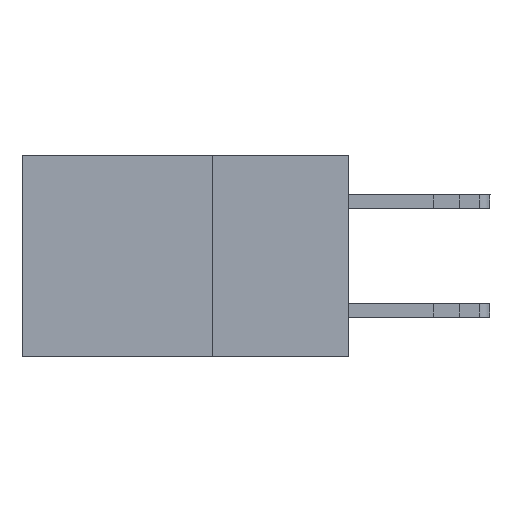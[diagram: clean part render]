
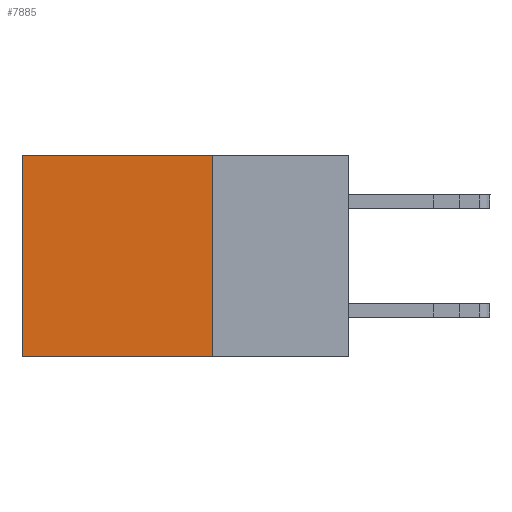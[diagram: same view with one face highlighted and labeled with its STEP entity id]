
A CAD part, left-side view. The second image highlights one B-rep face of the part: STEP entity #7885.
In plain terms, the highlighted planar face has unit normal (-1, 0, 0).
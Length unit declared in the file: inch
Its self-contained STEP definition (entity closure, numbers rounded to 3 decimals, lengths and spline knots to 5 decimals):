
#1 = CARTESIAN_POINT ( 'NONE',  ( 0.298, 0.6, 0. ) ) ;
#1360 = DIRECTION ( 'NONE',  ( 0., 0., -1. ) ) ;
#1648 = DIRECTION ( 'NONE',  ( 0., 0., -1. ) ) ;
#1945 = DIRECTION ( 'NONE',  ( 0., 0., -1. ) ) ;
#3186 = ORIENTED_EDGE ( 'NONE', *, *, #13528, .T. ) ;
#3212 = EDGE_CURVE ( 'NONE', #13332, #5409, #4690, .T. ) ;
#3219 = ORIENTED_EDGE ( 'NONE', *, *, #3212, .F. ) ;
#3785 = DIRECTION ( 'NONE',  ( 0., 1., 0. ) ) ;
#4531 = CARTESIAN_POINT ( 'NONE',  ( 0.298, 0.25, -0.37 ) ) ;
#4690 = LINE ( 'NONE', #11359, #9001 ) ;
#5409 = VERTEX_POINT ( 'NONE', #10916 ) ;
#6445 = CARTESIAN_POINT ( 'NONE',  ( 0.298, 0.6, 0. ) ) ;
#7378 = CARTESIAN_POINT ( 'NONE',  ( 0.298, 0.25, 0. ) ) ;
#7885 = ADVANCED_FACE ( 'NONE', ( #17855 ), #12615, .F. ) ;
#8250 = EDGE_LOOP ( 'NONE', ( #17135, #3219, #12923, #3186 ) ) ;
#8808 = VECTOR ( 'NONE', #1945, 39.37008 ) ;
#9001 = VECTOR ( 'NONE', #18022, 39.37008 ) ;
#9325 = EDGE_CURVE ( 'NONE', #12224, #13332, #16624, .T. ) ;
#10916 = CARTESIAN_POINT ( 'NONE',  ( 0.298, 0.6, -0.37 ) ) ;
#11359 = CARTESIAN_POINT ( 'NONE',  ( 0.298, 0.25, -0.37 ) ) ;
#11376 = CARTESIAN_POINT ( 'NONE',  ( 0.298, 0.25, 0. ) ) ;
#12224 = VERTEX_POINT ( 'NONE', #15563 ) ;
#12615 = PLANE ( 'NONE',  #15096 ) ;
#12923 = ORIENTED_EDGE ( 'NONE', *, *, #9325, .F. ) ;
#13332 = VERTEX_POINT ( 'NONE', #4531 ) ;
#13528 = EDGE_CURVE ( 'NONE', #12224, #17185, #19178, .T. ) ;
#13882 = VECTOR ( 'NONE', #3785, 39.37008 ) ;
#15096 = AXIS2_PLACEMENT_3D ( 'NONE', #19276, #17635, #1360 ) ;
#15563 = CARTESIAN_POINT ( 'NONE',  ( 0.298, 0.25, 0. ) ) ;
#16624 = LINE ( 'NONE', #11376, #19000 ) ;
#17135 = ORIENTED_EDGE ( 'NONE', *, *, #18582, .T. ) ;
#17185 = VERTEX_POINT ( 'NONE', #6445 ) ;
#17635 = DIRECTION ( 'NONE',  ( 1., 0., 0. ) ) ;
#17855 = FACE_OUTER_BOUND ( 'NONE', #8250, .T. ) ;
#18022 = DIRECTION ( 'NONE',  ( 0., 1., 0. ) ) ;
#18582 = EDGE_CURVE ( 'NONE', #17185, #5409, #20275, .T. ) ;
#19000 = VECTOR ( 'NONE', #1648, 39.37008 ) ;
#19178 = LINE ( 'NONE', #7378, #13882 ) ;
#19276 = CARTESIAN_POINT ( 'NONE',  ( 0.298, 0.25, 0. ) ) ;
#20275 = LINE ( 'NONE', #1, #8808 ) ;
